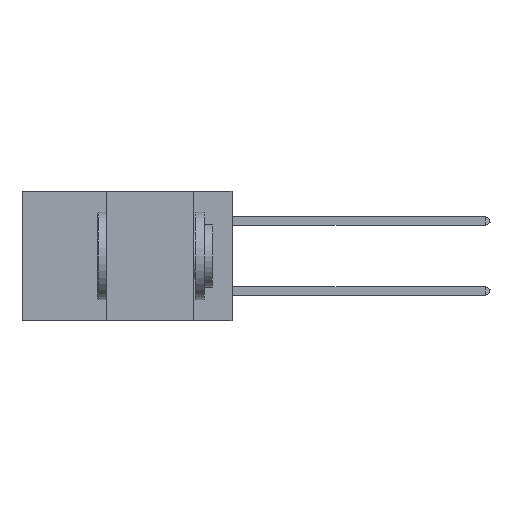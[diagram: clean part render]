
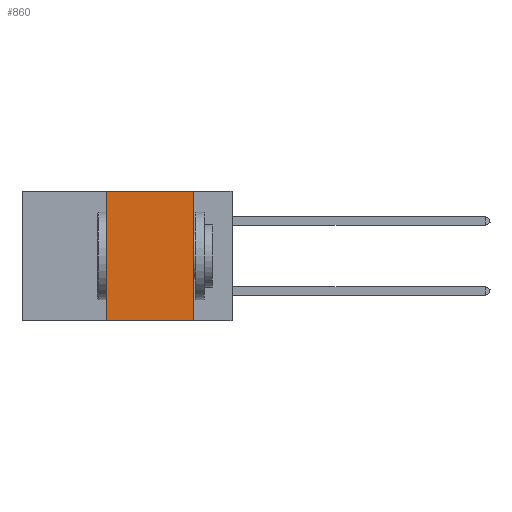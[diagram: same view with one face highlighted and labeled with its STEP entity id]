
A CAD part, left-side view. The second image highlights one B-rep face of the part: STEP entity #860.
In plain terms, the highlighted planar face has unit normal (-1, 0, 0).
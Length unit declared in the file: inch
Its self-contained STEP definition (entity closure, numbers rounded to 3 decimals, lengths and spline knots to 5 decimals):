
#471 = VECTOR ( 'NONE', #8514, 39.37008 ) ;
#512 = ORIENTED_EDGE ( 'NONE', *, *, #4160, .F. ) ;
#551 = ORIENTED_EDGE ( 'NONE', *, *, #7943, .F. ) ;
#614 = ORIENTED_EDGE ( 'NONE', *, *, #692, .F. ) ;
#692 = EDGE_CURVE ( 'NONE', #8327, #12176, #7581, .T. ) ;
#834 = ORIENTED_EDGE ( 'NONE', *, *, #11546, .T. ) ;
#860 = ADVANCED_FACE ( 'NONE', ( #10819 ), #11744, .F. ) ;
#1052 = VECTOR ( 'NONE', #2985, 39.37008 ) ;
#1712 = EDGE_LOOP ( 'NONE', ( #512, #551, #614, #834 ) ) ;
#2985 = DIRECTION ( 'NONE',  ( 0., -1., 0. ) ) ;
#3084 = LINE ( 'NONE', #12186, #5545 ) ;
#3202 = LINE ( 'NONE', #8549, #471 ) ;
#3281 = VERTEX_POINT ( 'NONE', #11862 ) ;
#3495 = LINE ( 'NONE', #8963, #1052 ) ;
#4160 = EDGE_CURVE ( 'NONE', #10854, #3281, #3202, .T. ) ;
#4606 = CARTESIAN_POINT ( 'NONE',  ( 0., 0.6, 0. ) ) ;
#4941 = VECTOR ( 'NONE', #10122, 39.37008 ) ;
#5545 = VECTOR ( 'NONE', #11251, 39.37008 ) ;
#7456 = CARTESIAN_POINT ( 'NONE',  ( 0., 0.36, 0. ) ) ;
#7581 = LINE ( 'NONE', #10712, #4941 ) ;
#7943 = EDGE_CURVE ( 'NONE', #12176, #10854, #3084, .T. ) ;
#8043 = CARTESIAN_POINT ( 'NONE',  ( 0., 0.36, -0.37 ) ) ;
#8327 = VERTEX_POINT ( 'NONE', #8043 ) ;
#8514 = DIRECTION ( 'NONE',  ( 0., 0., -1. ) ) ;
#8549 = CARTESIAN_POINT ( 'NONE',  ( 0., 0.11, 0. ) ) ;
#8963 = CARTESIAN_POINT ( 'NONE',  ( 0., 0.6, -0.37 ) ) ;
#9419 = AXIS2_PLACEMENT_3D ( 'NONE', #4606, #11299, #12446 ) ;
#10122 = DIRECTION ( 'NONE',  ( 0., 0., 1. ) ) ;
#10712 = CARTESIAN_POINT ( 'NONE',  ( 0., 0.36, 0. ) ) ;
#10819 = FACE_OUTER_BOUND ( 'NONE', #1712, .T. ) ;
#10854 = VERTEX_POINT ( 'NONE', #11656 ) ;
#11251 = DIRECTION ( 'NONE',  ( 0., -1., 0. ) ) ;
#11299 = DIRECTION ( 'NONE',  ( 1., 0., 0. ) ) ;
#11546 = EDGE_CURVE ( 'NONE', #8327, #3281, #3495, .T. ) ;
#11656 = CARTESIAN_POINT ( 'NONE',  ( 0., 0.11, 0. ) ) ;
#11744 = PLANE ( 'NONE',  #9419 ) ;
#11862 = CARTESIAN_POINT ( 'NONE',  ( 0., 0.11, -0.37 ) ) ;
#12176 = VERTEX_POINT ( 'NONE', #7456 ) ;
#12186 = CARTESIAN_POINT ( 'NONE',  ( 0., 0.6, 0. ) ) ;
#12446 = DIRECTION ( 'NONE',  ( 0., 0., -1. ) ) ;
